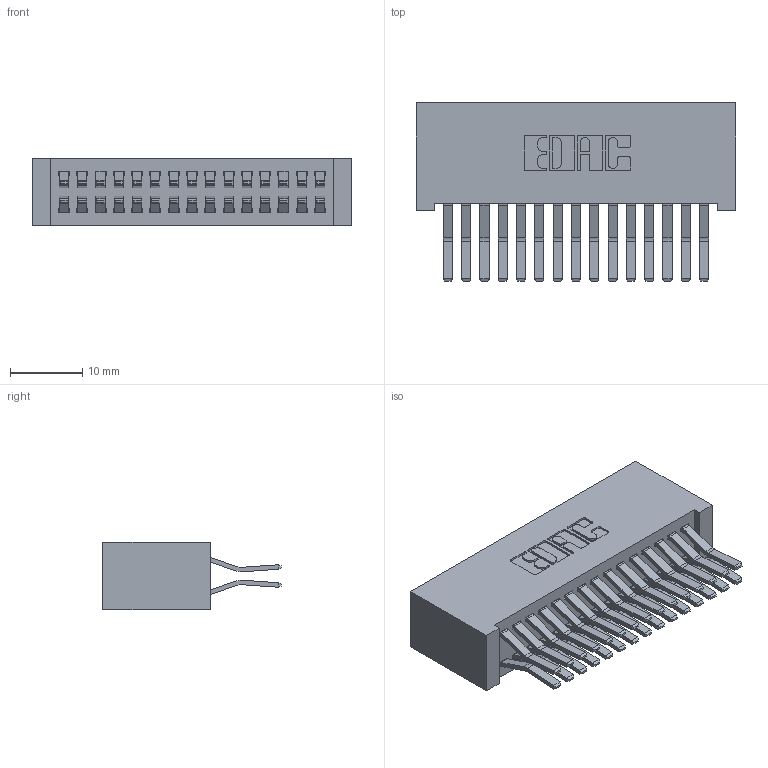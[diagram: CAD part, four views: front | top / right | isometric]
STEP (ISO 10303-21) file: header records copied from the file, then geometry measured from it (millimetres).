
FILE_DESCRIPTION (( 'STEP AP203' ), '1' );
FILE_NAME ('342-030-560-201.STEP', '2018-08-11T15:59:05', ( '' ), ( '' ), 'SwSTEP 2.0', 'SolidWorks 2016', '' );
FILE_SCHEMA (( 'CONFIG_CONTROL_DESIGN' ));
Length unit declared in the file: inch
Products named in the file (3): 345-292-001_560 Tail; 342-030-560-201; 342 Part_Lugless
Assembly tree (31 placements, depth 2):
  342-030-560-201
    342 Part_Lugless
    345-292-001_560 Tail  x30
Bounding box: 44.35 x 24.78 x 9.4 mm (x, y, z)
Volume: 4493.4 mm3; surface area: 7567.3 mm2
Topology: 31 solids, 31 shells, 1722 faces, 5105 edges, 3362 vertices
Faces by surface type: plane 1142, cylinder 580
Entity records: 12821 total; most frequent: CARTESIAN_POINT 2154, ORIENTED_EDGE 2090, DIRECTION 1885, EDGE_CURVE 1045, LINE 921, VECTOR 921, VERTEX_POINT 694, AXIS2_PLACEMENT_3D 482
